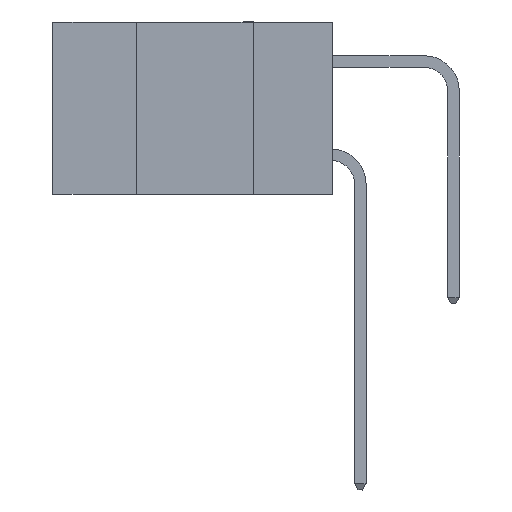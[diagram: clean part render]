
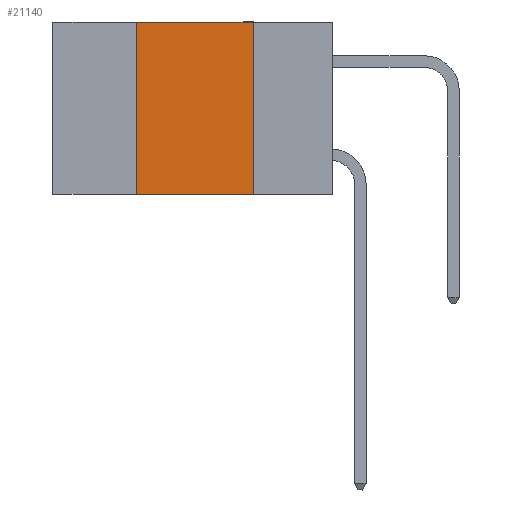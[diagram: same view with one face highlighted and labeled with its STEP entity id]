
A CAD part, left-side view. The second image highlights one B-rep face of the part: STEP entity #21140.
In plain terms, the highlighted planar face has unit normal (-1, 0, 0).
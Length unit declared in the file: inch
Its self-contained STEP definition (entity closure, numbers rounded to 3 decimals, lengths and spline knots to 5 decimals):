
#770 = LINE ( 'NONE', #8899, #8914 ) ;
#887 = AXIS2_PLACEMENT_3D ( 'NONE', #6975, #20461, #24274 ) ;
#2673 = LINE ( 'NONE', #7304, #19457 ) ;
#3363 = PLANE ( 'NONE',  #887 ) ;
#3446 = LINE ( 'NONE', #7777, #12121 ) ;
#6721 = CARTESIAN_POINT ( 'NONE',  ( 0., 0.17, -0.37 ) ) ;
#6877 = FACE_OUTER_BOUND ( 'NONE', #11145, .T. ) ;
#6975 = CARTESIAN_POINT ( 'NONE',  ( 0., 0.6, 0. ) ) ;
#7134 = DIRECTION ( 'NONE',  ( 0., -1., 0. ) ) ;
#7304 = CARTESIAN_POINT ( 'NONE',  ( 0., 0.42, 0. ) ) ;
#7707 = VERTEX_POINT ( 'NONE', #6721 ) ;
#7777 = CARTESIAN_POINT ( 'NONE',  ( 0., 0.17, 0. ) ) ;
#7851 = EDGE_CURVE ( 'NONE', #20335, #17073, #770, .T. ) ;
#7947 = DIRECTION ( 'NONE',  ( 0., 0., -1. ) ) ;
#8899 = CARTESIAN_POINT ( 'NONE',  ( 0., 0.6, 0. ) ) ;
#8914 = VECTOR ( 'NONE', #7134, 39.37008 ) ;
#9100 = CARTESIAN_POINT ( 'NONE',  ( 0., 0.17, 0. ) ) ;
#9755 = CARTESIAN_POINT ( 'NONE',  ( 0., 0.42, 0. ) ) ;
#9811 = DIRECTION ( 'NONE',  ( 0., -1., 0. ) ) ;
#11145 = EDGE_LOOP ( 'NONE', ( #15388, #21575, #14932, #18165 ) ) ;
#11895 = VECTOR ( 'NONE', #9811, 39.37008 ) ;
#12121 = VECTOR ( 'NONE', #7947, 39.37008 ) ;
#12918 = EDGE_CURVE ( 'NONE', #17077, #20335, #2673, .T. ) ;
#13678 = EDGE_CURVE ( 'NONE', #17077, #7707, #22134, .T. ) ;
#14932 = ORIENTED_EDGE ( 'NONE', *, *, #12918, .F. ) ;
#15388 = ORIENTED_EDGE ( 'NONE', *, *, #23690, .F. ) ;
#16517 = DIRECTION ( 'NONE',  ( 0., 0., 1. ) ) ;
#17073 = VERTEX_POINT ( 'NONE', #9100 ) ;
#17077 = VERTEX_POINT ( 'NONE', #20358 ) ;
#18165 = ORIENTED_EDGE ( 'NONE', *, *, #13678, .T. ) ;
#19457 = VECTOR ( 'NONE', #16517, 39.37008 ) ;
#20335 = VERTEX_POINT ( 'NONE', #9755 ) ;
#20358 = CARTESIAN_POINT ( 'NONE',  ( 0., 0.42, -0.37 ) ) ;
#20461 = DIRECTION ( 'NONE',  ( 1., 0., 0. ) ) ;
#21140 = ADVANCED_FACE ( 'NONE', ( #6877 ), #3363, .F. ) ;
#21575 = ORIENTED_EDGE ( 'NONE', *, *, #7851, .F. ) ;
#21986 = CARTESIAN_POINT ( 'NONE',  ( 0., 0.6, -0.37 ) ) ;
#22134 = LINE ( 'NONE', #21986, #11895 ) ;
#23690 = EDGE_CURVE ( 'NONE', #17073, #7707, #3446, .T. ) ;
#24274 = DIRECTION ( 'NONE',  ( 0., 0., -1. ) ) ;
